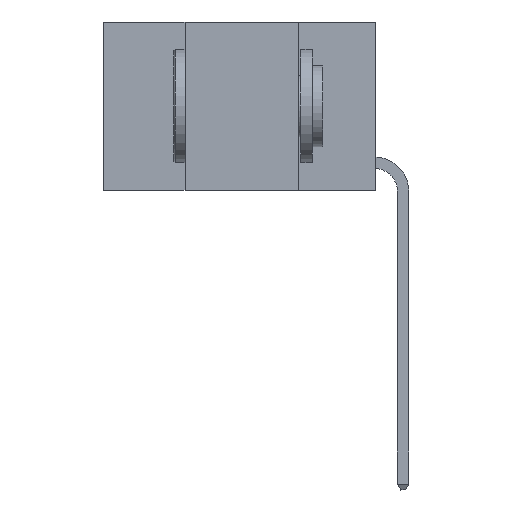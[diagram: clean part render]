
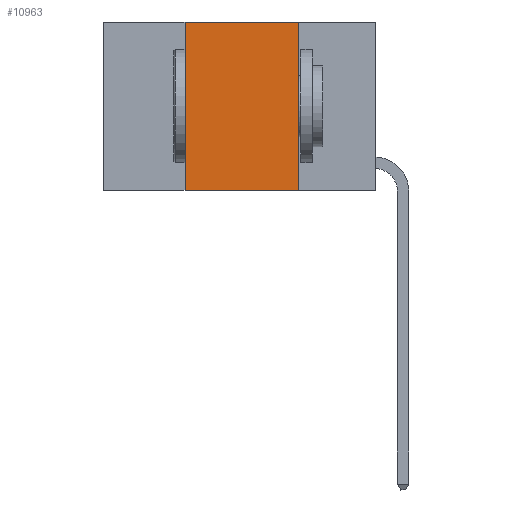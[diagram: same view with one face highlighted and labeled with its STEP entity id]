
A CAD part, left-side view. The second image highlights one B-rep face of the part: STEP entity #10963.
In plain terms, the highlighted planar face has unit normal (-1, 0, 0).
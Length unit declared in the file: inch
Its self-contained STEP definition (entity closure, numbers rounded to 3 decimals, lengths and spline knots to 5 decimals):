
#254 = ORIENTED_EDGE ( 'NONE', *, *, #10970, .F. ) ;
#329 = EDGE_LOOP ( 'NONE', ( #3865, #4338, #254, #9936 ) ) ;
#457 = EDGE_CURVE ( 'NONE', #9508, #10163, #10088, .T. ) ;
#970 = CARTESIAN_POINT ( 'NONE',  ( 0., 0.6, 0. ) ) ;
#1419 = DIRECTION ( 'NONE',  ( 1., 0., 0. ) ) ;
#1485 = DIRECTION ( 'NONE',  ( 0., 0., 1. ) ) ;
#2459 = CARTESIAN_POINT ( 'NONE',  ( 0., 0.6, -0.37 ) ) ;
#2543 = CARTESIAN_POINT ( 'NONE',  ( 0., 0.42, 0. ) ) ;
#2772 = VERTEX_POINT ( 'NONE', #6139 ) ;
#3366 = FACE_OUTER_BOUND ( 'NONE', #329, .T. ) ;
#3865 = ORIENTED_EDGE ( 'NONE', *, *, #12974, .F. ) ;
#4338 = ORIENTED_EDGE ( 'NONE', *, *, #6603, .F. ) ;
#5371 = VECTOR ( 'NONE', #9155, 39.37008 ) ;
#5436 = DIRECTION ( 'NONE',  ( 0., 0., -1. ) ) ;
#6139 = CARTESIAN_POINT ( 'NONE',  ( 0., 0.17, 0. ) ) ;
#6603 = EDGE_CURVE ( 'NONE', #10666, #2772, #12585, .T. ) ;
#6680 = VECTOR ( 'NONE', #6892, 39.37008 ) ;
#6892 = DIRECTION ( 'NONE',  ( 0., -1., 0. ) ) ;
#7979 = DIRECTION ( 'NONE',  ( 0., 0., -1. ) ) ;
#8036 = CARTESIAN_POINT ( 'NONE',  ( 0., 0.17, -0.37 ) ) ;
#8791 = AXIS2_PLACEMENT_3D ( 'NONE', #8848, #1419, #5436 ) ;
#8848 = CARTESIAN_POINT ( 'NONE',  ( 0., 0.6, 0. ) ) ;
#8948 = LINE ( 'NONE', #12256, #10574 ) ;
#9155 = DIRECTION ( 'NONE',  ( 0., -1., 0. ) ) ;
#9508 = VERTEX_POINT ( 'NONE', #11695 ) ;
#9936 = ORIENTED_EDGE ( 'NONE', *, *, #457, .T. ) ;
#10088 = LINE ( 'NONE', #2459, #6680 ) ;
#10163 = VERTEX_POINT ( 'NONE', #8036 ) ;
#10574 = VECTOR ( 'NONE', #7979, 39.37008 ) ;
#10666 = VERTEX_POINT ( 'NONE', #11162 ) ;
#10963 = ADVANCED_FACE ( 'NONE', ( #3366 ), #12081, .F. ) ;
#10970 = EDGE_CURVE ( 'NONE', #9508, #10666, #13137, .T. ) ;
#11162 = CARTESIAN_POINT ( 'NONE',  ( 0., 0.42, 0. ) ) ;
#11464 = VECTOR ( 'NONE', #1485, 39.37008 ) ;
#11695 = CARTESIAN_POINT ( 'NONE',  ( 0., 0.42, -0.37 ) ) ;
#12081 = PLANE ( 'NONE',  #8791 ) ;
#12256 = CARTESIAN_POINT ( 'NONE',  ( 0., 0.17, 0. ) ) ;
#12585 = LINE ( 'NONE', #970, #5371 ) ;
#12974 = EDGE_CURVE ( 'NONE', #2772, #10163, #8948, .T. ) ;
#13137 = LINE ( 'NONE', #2543, #11464 ) ;
